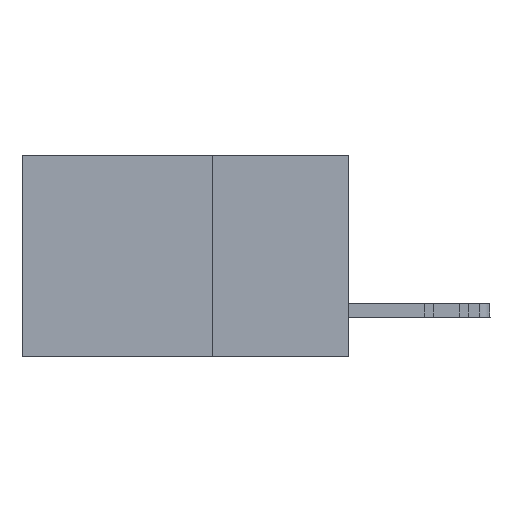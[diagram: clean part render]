
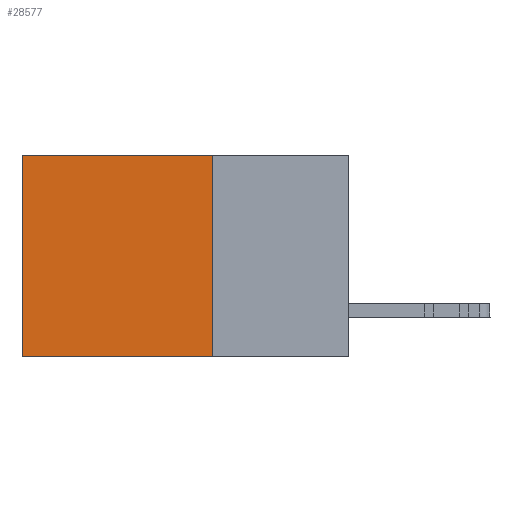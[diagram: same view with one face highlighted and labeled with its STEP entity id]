
A CAD part, left-side view. The second image highlights one B-rep face of the part: STEP entity #28577.
In plain terms, the highlighted planar face has unit normal (-1, 0, 0).
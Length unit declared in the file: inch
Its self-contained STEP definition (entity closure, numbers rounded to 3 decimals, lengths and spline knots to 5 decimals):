
#1301 = VERTEX_POINT ( 'NONE', #20424 ) ;
#2699 = CARTESIAN_POINT ( 'NONE',  ( 0.298, 0.25, 0. ) ) ;
#3233 = CARTESIAN_POINT ( 'NONE',  ( 0.298, 0.6, -0.37 ) ) ;
#4232 = VERTEX_POINT ( 'NONE', #15480 ) ;
#5313 = EDGE_LOOP ( 'NONE', ( #28912, #7244, #21392, #21996 ) ) ;
#6118 = DIRECTION ( 'NONE',  ( 0., 0., -1. ) ) ;
#6762 = FACE_OUTER_BOUND ( 'NONE', #5313, .T. ) ;
#7244 = ORIENTED_EDGE ( 'NONE', *, *, #25670, .F. ) ;
#7860 = DIRECTION ( 'NONE',  ( 0., 1., 0. ) ) ;
#8997 = CARTESIAN_POINT ( 'NONE',  ( 0.298, 0.25, 0. ) ) ;
#9179 = PLANE ( 'NONE',  #14178 ) ;
#9326 = VECTOR ( 'NONE', #18941, 39.37008 ) ;
#9332 = VECTOR ( 'NONE', #6118, 39.37008 ) ;
#10476 = EDGE_CURVE ( 'NONE', #26687, #13214, #31159, .T. ) ;
#13198 = CARTESIAN_POINT ( 'NONE',  ( 0.298, 0.6, 0. ) ) ;
#13214 = VERTEX_POINT ( 'NONE', #3233 ) ;
#13342 = DIRECTION ( 'NONE',  ( 0., 1., 0. ) ) ;
#14178 = AXIS2_PLACEMENT_3D ( 'NONE', #21544, #18977, #26965 ) ;
#15480 = CARTESIAN_POINT ( 'NONE',  ( 0.298, 0.25, -0.37 ) ) ;
#16190 = VECTOR ( 'NONE', #13342, 39.37008 ) ;
#16229 = CARTESIAN_POINT ( 'NONE',  ( 0.298, 0.25, -0.37 ) ) ;
#18632 = LINE ( 'NONE', #16229, #16190 ) ;
#18941 = DIRECTION ( 'NONE',  ( 0., 0., -1. ) ) ;
#18977 = DIRECTION ( 'NONE',  ( 1., 0., 0. ) ) ;
#20393 = LINE ( 'NONE', #2699, #29085 ) ;
#20424 = CARTESIAN_POINT ( 'NONE',  ( 0.298, 0.25, 0. ) ) ;
#21392 = ORIENTED_EDGE ( 'NONE', *, *, #21692, .F. ) ;
#21544 = CARTESIAN_POINT ( 'NONE',  ( 0.298, 0.25, 0. ) ) ;
#21692 = EDGE_CURVE ( 'NONE', #1301, #4232, #26037, .T. ) ;
#21996 = ORIENTED_EDGE ( 'NONE', *, *, #27191, .T. ) ;
#25670 = EDGE_CURVE ( 'NONE', #4232, #13214, #18632, .T. ) ;
#26037 = LINE ( 'NONE', #8997, #9332 ) ;
#26687 = VERTEX_POINT ( 'NONE', #13198 ) ;
#26965 = DIRECTION ( 'NONE',  ( 0., 0., -1. ) ) ;
#27191 = EDGE_CURVE ( 'NONE', #1301, #26687, #20393, .T. ) ;
#28577 = ADVANCED_FACE ( 'NONE', ( #6762 ), #9179, .F. ) ;
#28912 = ORIENTED_EDGE ( 'NONE', *, *, #10476, .T. ) ;
#29085 = VECTOR ( 'NONE', #7860, 39.37008 ) ;
#31159 = LINE ( 'NONE', #31477, #9326 ) ;
#31477 = CARTESIAN_POINT ( 'NONE',  ( 0.298, 0.6, 0. ) ) ;
